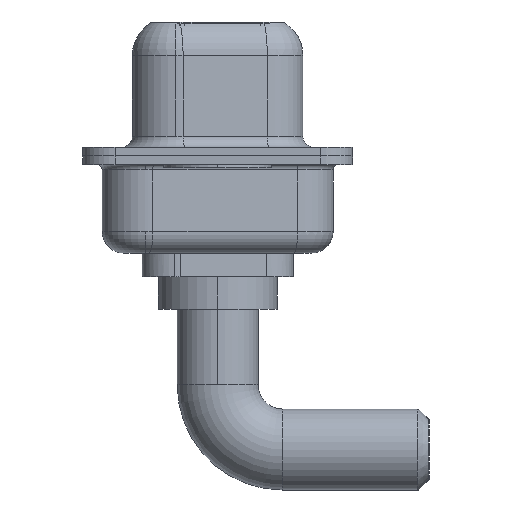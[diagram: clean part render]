
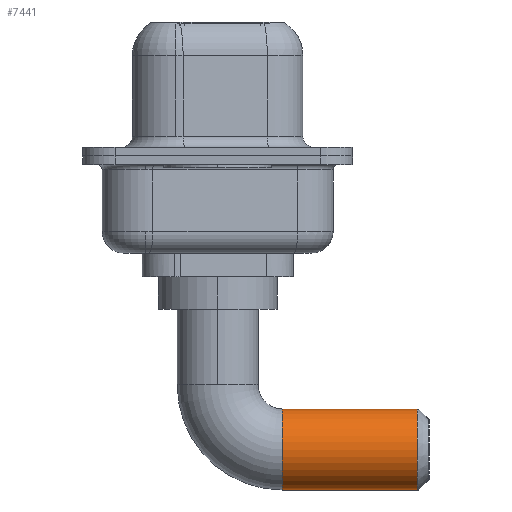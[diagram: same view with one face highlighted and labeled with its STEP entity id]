
A CAD part, left-side view. The second image highlights one B-rep face of the part: STEP entity #7441.
In plain terms, the highlighted cylindrical face has radius 1.875 mm (diameter 3.75 mm), a partial arc.
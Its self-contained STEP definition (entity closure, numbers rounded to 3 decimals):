
#73 = LINE ( 'NONE', #11181, #3865 ) ;
#470 = CARTESIAN_POINT ( 'NONE',  ( 0., -3., -4.625 ) ) ;
#529 = DIRECTION ( 'NONE',  ( 0., 1., 0. ) ) ;
#1139 = EDGE_CURVE ( 'NONE', #4766, #8382, #7587, .T. ) ;
#1596 = CARTESIAN_POINT ( 'NONE',  ( 0., -3., -8.375 ) ) ;
#1980 = EDGE_CURVE ( 'NONE', #6382, #7385, #2196, .T. ) ;
#2196 = CIRCLE ( 'NONE', #10126, 1.875 ) ;
#2510 = FACE_OUTER_BOUND ( 'NONE', #10044, .T. ) ;
#2875 = DIRECTION ( 'NONE',  ( 0., -1., 0. ) ) ;
#3022 = DIRECTION ( 'NONE',  ( 0., -1., 0. ) ) ;
#3179 = ORIENTED_EDGE ( 'NONE', *, *, #1139, .T. ) ;
#3224 = VECTOR ( 'NONE', #6013, 1000. ) ;
#3242 = CYLINDRICAL_SURFACE ( 'NONE', #9653, 1.875 ) ;
#3310 = DIRECTION ( 'NONE',  ( 0., -1., 0. ) ) ;
#3865 = VECTOR ( 'NONE', #2875, 1000. ) ;
#4201 = CARTESIAN_POINT ( 'NONE',  ( 0., -3., -6.5 ) ) ;
#4236 = DIRECTION ( 'NONE',  ( 0., 0., -1. ) ) ;
#4766 = VERTEX_POINT ( 'NONE', #9018 ) ;
#5017 = CARTESIAN_POINT ( 'NONE',  ( 0., -9.25, -6.5 ) ) ;
#5096 = DIRECTION ( 'NONE',  ( 0., 0., -1. ) ) ;
#5910 = EDGE_CURVE ( 'NONE', #6382, #8382, #73, .T. ) ;
#6013 = DIRECTION ( 'NONE',  ( 0., -1., 0. ) ) ;
#6382 = VERTEX_POINT ( 'NONE', #470 ) ;
#7385 = VERTEX_POINT ( 'NONE', #1596 ) ;
#7441 = ADVANCED_FACE ( 'NONE', ( #2510 ), #3242, .T. ) ;
#7587 = CIRCLE ( 'NONE', #8748, 1.875 ) ;
#7837 = LINE ( 'NONE', #11550, #3224 ) ;
#8269 = ORIENTED_EDGE ( 'NONE', *, *, #5910, .F. ) ;
#8382 = VERTEX_POINT ( 'NONE', #9013 ) ;
#8748 = AXIS2_PLACEMENT_3D ( 'NONE', #5017, #529, #4236 ) ;
#9013 = CARTESIAN_POINT ( 'NONE',  ( 0., -9.25, -4.625 ) ) ;
#9018 = CARTESIAN_POINT ( 'NONE',  ( 0., -9.25, -8.375 ) ) ;
#9493 = CARTESIAN_POINT ( 'NONE',  ( 0., -3., -6.5 ) ) ;
#9617 = DIRECTION ( 'NONE',  ( -1., 0., 0. ) ) ;
#9653 = AXIS2_PLACEMENT_3D ( 'NONE', #4201, #3310, #5096 ) ;
#10013 = EDGE_CURVE ( 'NONE', #7385, #4766, #7837, .T. ) ;
#10044 = EDGE_LOOP ( 'NONE', ( #8269, #11112, #11816, #3179 ) ) ;
#10126 = AXIS2_PLACEMENT_3D ( 'NONE', #9493, #3022, #9617 ) ;
#11112 = ORIENTED_EDGE ( 'NONE', *, *, #1980, .T. ) ;
#11181 = CARTESIAN_POINT ( 'NONE',  ( 0., -3., -4.625 ) ) ;
#11550 = CARTESIAN_POINT ( 'NONE',  ( 0., -3., -8.375 ) ) ;
#11816 = ORIENTED_EDGE ( 'NONE', *, *, #10013, .T. ) ;
